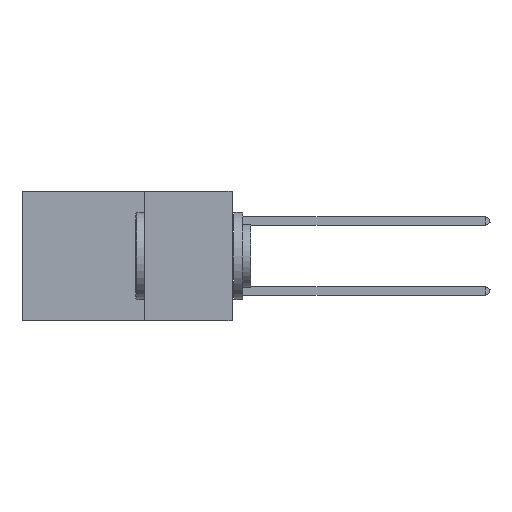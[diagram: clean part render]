
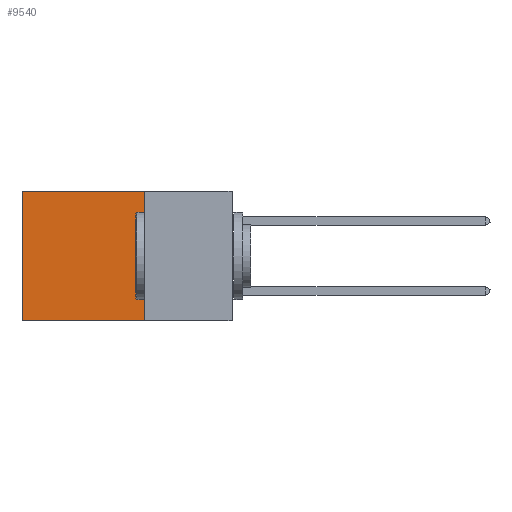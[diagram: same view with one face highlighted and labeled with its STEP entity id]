
A CAD part, left-side view. The second image highlights one B-rep face of the part: STEP entity #9540.
In plain terms, the highlighted planar face has unit normal (-1, 0, 0).
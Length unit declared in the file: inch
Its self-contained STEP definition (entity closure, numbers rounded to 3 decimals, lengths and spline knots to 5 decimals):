
#594 = LINE ( 'NONE', #22804, #24052 ) ;
#1025 = LINE ( 'NONE', #11160, #20767 ) ;
#1941 = DIRECTION ( 'NONE',  ( 0., 0., -1. ) ) ;
#3905 = ORIENTED_EDGE ( 'NONE', *, *, #11374, .F. ) ;
#5295 = DIRECTION ( 'NONE',  ( 1., 0., 0. ) ) ;
#7916 = AXIS2_PLACEMENT_3D ( 'NONE', #11826, #5295, #26243 ) ;
#9540 = ADVANCED_FACE ( 'NONE', ( #22718 ), #11294, .F. ) ;
#10635 = EDGE_CURVE ( 'NONE', #24812, #33498, #15661, .T. ) ;
#11160 = CARTESIAN_POINT ( 'NONE',  ( 0.2875, 0.25, -0.37 ) ) ;
#11294 = PLANE ( 'NONE',  #7916 ) ;
#11374 = EDGE_CURVE ( 'NONE', #37306, #17831, #1025, .T. ) ;
#11473 = CARTESIAN_POINT ( 'NONE',  ( 0.2875, 0.6, 0. ) ) ;
#11826 = CARTESIAN_POINT ( 'NONE',  ( 0.2875, 0.25, 0. ) ) ;
#13566 = CARTESIAN_POINT ( 'NONE',  ( 0.2875, 0.25, 0. ) ) ;
#15661 = LINE ( 'NONE', #13566, #24057 ) ;
#16660 = CARTESIAN_POINT ( 'NONE',  ( 0.2875, 0.25, -0.37 ) ) ;
#17831 = VERTEX_POINT ( 'NONE', #34523 ) ;
#20531 = CARTESIAN_POINT ( 'NONE',  ( 0.2875, 0.6, 0. ) ) ;
#20767 = VECTOR ( 'NONE', #23622, 39.37008 ) ;
#21702 = ORIENTED_EDGE ( 'NONE', *, *, #30424, .T. ) ;
#22718 = FACE_OUTER_BOUND ( 'NONE', #26061, .T. ) ;
#22804 = CARTESIAN_POINT ( 'NONE',  ( 0.2875, 0.25, 0. ) ) ;
#23006 = DIRECTION ( 'NONE',  ( 0., 0., -1. ) ) ;
#23058 = ORIENTED_EDGE ( 'NONE', *, *, #29649, .F. ) ;
#23622 = DIRECTION ( 'NONE',  ( 0., 1., 0. ) ) ;
#24052 = VECTOR ( 'NONE', #1941, 39.37008 ) ;
#24057 = VECTOR ( 'NONE', #37593, 39.37008 ) ;
#24812 = VERTEX_POINT ( 'NONE', #26683 ) ;
#26061 = EDGE_LOOP ( 'NONE', ( #21702, #3905, #23058, #30960 ) ) ;
#26243 = DIRECTION ( 'NONE',  ( 0., 0., -1. ) ) ;
#26683 = CARTESIAN_POINT ( 'NONE',  ( 0.2875, 0.25, 0. ) ) ;
#29649 = EDGE_CURVE ( 'NONE', #24812, #37306, #594, .T. ) ;
#30424 = EDGE_CURVE ( 'NONE', #33498, #17831, #32006, .T. ) ;
#30960 = ORIENTED_EDGE ( 'NONE', *, *, #10635, .T. ) ;
#32006 = LINE ( 'NONE', #20531, #37132 ) ;
#33498 = VERTEX_POINT ( 'NONE', #11473 ) ;
#34523 = CARTESIAN_POINT ( 'NONE',  ( 0.2875, 0.6, -0.37 ) ) ;
#37132 = VECTOR ( 'NONE', #23006, 39.37008 ) ;
#37306 = VERTEX_POINT ( 'NONE', #16660 ) ;
#37593 = DIRECTION ( 'NONE',  ( 0., 1., 0. ) ) ;
